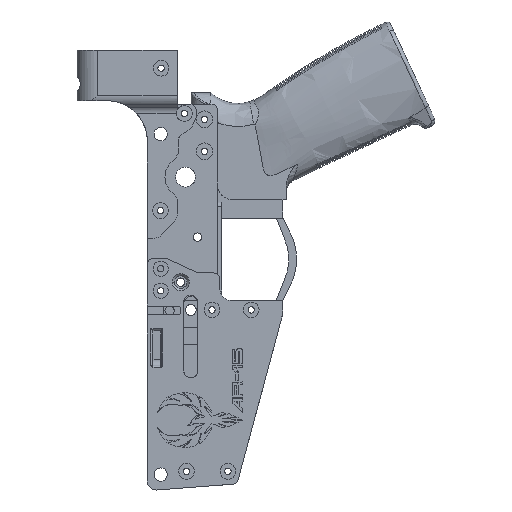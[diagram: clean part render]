
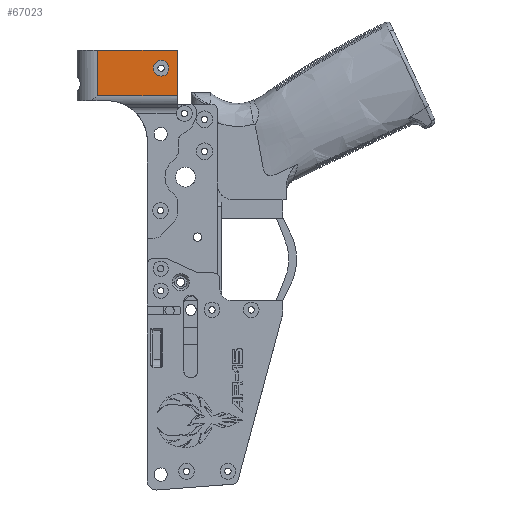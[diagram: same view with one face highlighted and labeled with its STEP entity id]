
A CAD part, left-side view. The second image highlights one B-rep face of the part: STEP entity #67023.
In plain terms, the highlighted planar face has unit normal (-1, 0, 0).
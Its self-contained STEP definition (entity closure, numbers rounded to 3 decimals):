
#368 = DIRECTION ( 'NONE',  ( 1., 0., 0. ) ) ;
#6750 = CARTESIAN_POINT ( 'NONE',  ( -25., 7.678, 11.224 ) ) ;
#14213 = VECTOR ( 'NONE', #26167, 1000. ) ;
#15213 = VERTEX_POINT ( 'NONE', #75529 ) ;
#16472 = CARTESIAN_POINT ( 'NONE',  ( -25., -22.502, 2.734 ) ) ;
#17816 = VERTEX_POINT ( 'NONE', #130054 ) ;
#18314 = CARTESIAN_POINT ( 'NONE',  ( -25., -36.779, -10.291 ) ) ;
#22324 = DIRECTION ( 'NONE',  ( 0., 0., -1. ) ) ;
#23908 = VERTEX_POINT ( 'NONE', #6750 ) ;
#26167 = DIRECTION ( 'NONE',  ( 0., 0., 1. ) ) ;
#26538 = EDGE_CURVE ( 'NONE', #17816, #15213, #115380, .T. ) ;
#29956 = CIRCLE ( 'NONE', #32188, 3.75 ) ;
#30927 = CARTESIAN_POINT ( 'NONE',  ( -25., 7.678, -12.776 ) ) ;
#32188 = AXIS2_PLACEMENT_3D ( 'NONE', #45524, #110711, #121346 ) ;
#37696 = DIRECTION ( 'NONE',  ( -1., 0., 0. ) ) ;
#44564 = EDGE_CURVE ( 'NONE', #23908, #58409, #70827, .T. ) ;
#45524 = CARTESIAN_POINT ( 'NONE',  ( -25., -22.502, 2.734 ) ) ;
#47622 = DIRECTION ( 'NONE',  ( 0., 0., 1. ) ) ;
#48776 = CARTESIAN_POINT ( 'NONE',  ( -25., -30.202, -10.291 ) ) ;
#54295 = AXIS2_PLACEMENT_3D ( 'NONE', #16472, #37696, #47622 ) ;
#55754 = VERTEX_POINT ( 'NONE', #48776 ) ;
#56927 = EDGE_CURVE ( 'NONE', #58409, #55754, #72142, .T. ) ;
#56929 = DIRECTION ( 'NONE',  ( 0., 1., 0. ) ) ;
#57229 = ORIENTED_EDGE ( 'NONE', *, *, #56927, .T. ) ;
#58065 = LINE ( 'NONE', #81415, #14213 ) ;
#58307 = AXIS2_PLACEMENT_3D ( 'NONE', #85406, #368, #22324 ) ;
#58409 = VERTEX_POINT ( 'NONE', #100267 ) ;
#59476 = EDGE_LOOP ( 'NONE', ( #136873, #57229, #80709, #109859 ) ) ;
#67023 = ADVANCED_FACE ( 'NONE', ( #130742, #88207 ), #74783, .F. ) ;
#70827 = LINE ( 'NONE', #30927, #117703 ) ;
#72142 = LINE ( 'NONE', #18314, #79649 ) ;
#73839 = EDGE_CURVE ( 'NONE', #81964, #23908, #78176, .T. ) ;
#74783 = PLANE ( 'NONE',  #58307 ) ;
#75529 = CARTESIAN_POINT ( 'NONE',  ( -25., -22.502, -1.016 ) ) ;
#78176 = LINE ( 'NONE', #131359, #120093 ) ;
#79649 = VECTOR ( 'NONE', #125326, 1000. ) ;
#79725 = EDGE_CURVE ( 'NONE', #55754, #81964, #58065, .T. ) ;
#80709 = ORIENTED_EDGE ( 'NONE', *, *, #79725, .T. ) ;
#81415 = CARTESIAN_POINT ( 'NONE',  ( -25., -30.202, -14.306 ) ) ;
#81964 = VERTEX_POINT ( 'NONE', #110650 ) ;
#85406 = CARTESIAN_POINT ( 'NONE',  ( -25., -36.779, -288600.29 ) ) ;
#88207 = FACE_OUTER_BOUND ( 'NONE', #59476, .T. ) ;
#96451 = EDGE_CURVE ( 'NONE', #15213, #17816, #29956, .T. ) ;
#100267 = CARTESIAN_POINT ( 'NONE',  ( -25., 7.678, -10.291 ) ) ;
#109859 = ORIENTED_EDGE ( 'NONE', *, *, #73839, .T. ) ;
#110650 = CARTESIAN_POINT ( 'NONE',  ( -25., -30.202, 11.224 ) ) ;
#110711 = DIRECTION ( 'NONE',  ( -1., 0., 0. ) ) ;
#111038 = EDGE_LOOP ( 'NONE', ( #114690, #116592 ) ) ;
#114049 = DIRECTION ( 'NONE',  ( 0., 0., -1. ) ) ;
#114690 = ORIENTED_EDGE ( 'NONE', *, *, #26538, .F. ) ;
#115380 = CIRCLE ( 'NONE', #54295, 3.75 ) ;
#116592 = ORIENTED_EDGE ( 'NONE', *, *, #96451, .F. ) ;
#117703 = VECTOR ( 'NONE', #114049, 1000. ) ;
#120093 = VECTOR ( 'NONE', #56929, 1000. ) ;
#121346 = DIRECTION ( 'NONE',  ( 0., 0., 1. ) ) ;
#125326 = DIRECTION ( 'NONE',  ( 0., -1., 0. ) ) ;
#130054 = CARTESIAN_POINT ( 'NONE',  ( -25., -22.502, 6.484 ) ) ;
#130742 = FACE_BOUND ( 'NONE', #111038, .T. ) ;
#131359 = CARTESIAN_POINT ( 'NONE',  ( -25., -36.779, 11.224 ) ) ;
#136873 = ORIENTED_EDGE ( 'NONE', *, *, #44564, .T. ) ;
